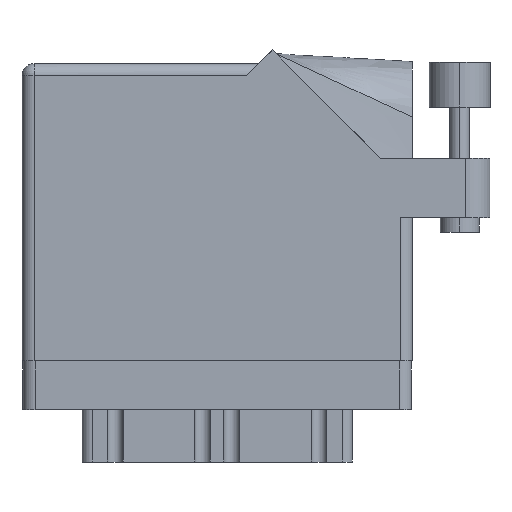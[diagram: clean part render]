
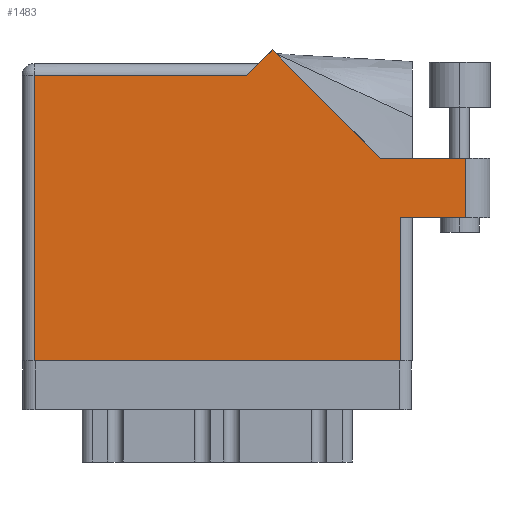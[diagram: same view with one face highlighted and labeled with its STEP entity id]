
A CAD part, front view. The second image highlights one B-rep face of the part: STEP entity #1483.
In plain terms, the highlighted face is planar.
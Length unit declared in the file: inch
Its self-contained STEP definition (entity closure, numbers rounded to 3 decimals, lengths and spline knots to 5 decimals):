
#313 = ORIENTED_EDGE ( 'NONE', *, *, #32996, .T. ) ;
#760 = CARTESIAN_POINT ( 'NONE',  ( 2.41, 1.044, 0. ) ) ;
#932 = VERTEX_POINT ( 'NONE', #34504 ) ;
#1483 = ADVANCED_FACE ( 'NONE', ( #16268 ), #7638, .F. ) ;
#1508 = CARTESIAN_POINT ( 'NONE',  ( 0., 1.468, 0. ) ) ;
#2046 = CARTESIAN_POINT ( 'NONE',  ( 0.062, 0., 0. ) ) ;
#2494 = CARTESIAN_POINT ( 'NONE',  ( 2.01, 0.737, 0. ) ) ;
#2505 = EDGE_LOOP ( 'NONE', ( #14980, #20236, #18831, #3973, #25659, #313, #23713, #31068, #27965 ) ) ;
#3094 = CARTESIAN_POINT ( 'NONE',  ( 1.155, 1.468, 0. ) ) ;
#3973 = ORIENTED_EDGE ( 'NONE', *, *, #20785, .T. ) ;
#4263 = DIRECTION ( 'NONE',  ( 0., 1., 0. ) ) ;
#4968 = LINE ( 'NONE', #2046, #15368 ) ;
#6280 = VECTOR ( 'NONE', #18075, 39.37008 ) ;
#6432 = VECTOR ( 'NONE', #33864, 39.37008 ) ;
#7322 = CARTESIAN_POINT ( 'NONE',  ( 1.948, 0., 0. ) ) ;
#7638 = PLANE ( 'NONE',  #19010 ) ;
#9730 = EDGE_CURVE ( 'NONE', #15255, #17082, #21563, .T. ) ;
#10452 = CARTESIAN_POINT ( 'NONE',  ( 0.062, 1.468, 0. ) ) ;
#10572 = DIRECTION ( 'NONE',  ( -1., 0., 0. ) ) ;
#10894 = VERTEX_POINT ( 'NONE', #10452 ) ;
#11469 = VERTEX_POINT ( 'NONE', #3094 ) ;
#11742 = VECTOR ( 'NONE', #31262, 39.37008 ) ;
#11778 = LINE ( 'NONE', #11996, #6280 ) ;
#11996 = CARTESIAN_POINT ( 'NONE',  ( 1.217, 1.53, 0. ) ) ;
#12164 = EDGE_CURVE ( 'NONE', #10894, #14437, #4968, .T. ) ;
#12780 = VERTEX_POINT ( 'NONE', #24798 ) ;
#12906 = EDGE_CURVE ( 'NONE', #12954, #932, #28499, .T. ) ;
#12954 = VERTEX_POINT ( 'NONE', #7322 ) ;
#14254 = CARTESIAN_POINT ( 'NONE',  ( 1.84442, 1.044, 0. ) ) ;
#14437 = VERTEX_POINT ( 'NONE', #14606 ) ;
#14606 = CARTESIAN_POINT ( 'NONE',  ( 0.062, 0., 0. ) ) ;
#14980 = ORIENTED_EDGE ( 'NONE', *, *, #23627, .T. ) ;
#15255 = VERTEX_POINT ( 'NONE', #27231 ) ;
#15368 = VECTOR ( 'NONE', #16556, 39.37008 ) ;
#15943 = EDGE_CURVE ( 'NONE', #12780, #11469, #11778, .T. ) ;
#16048 = CARTESIAN_POINT ( 'NONE',  ( 2.285, 1.044, 0. ) ) ;
#16268 = FACE_OUTER_BOUND ( 'NONE', #2505, .T. ) ;
#16556 = DIRECTION ( 'NONE',  ( 0., -1., 0. ) ) ;
#17082 = VERTEX_POINT ( 'NONE', #32617 ) ;
#18012 = EDGE_CURVE ( 'NONE', #14437, #12954, #22919, .T. ) ;
#18075 = DIRECTION ( 'NONE',  ( -0.707, -0.707, 0. ) ) ;
#18141 = VECTOR ( 'NONE', #4263, 39.37008 ) ;
#18784 = LINE ( 'NONE', #760, #23560 ) ;
#18831 = ORIENTED_EDGE ( 'NONE', *, *, #26727, .T. ) ;
#19010 = AXIS2_PLACEMENT_3D ( 'NONE', #19623, #28229, #10572 ) ;
#19623 = CARTESIAN_POINT ( 'NONE',  ( 0., 1.53, 0. ) ) ;
#19627 = VERTEX_POINT ( 'NONE', #14254 ) ;
#19886 = LINE ( 'NONE', #20094, #30640 ) ;
#20094 = CARTESIAN_POINT ( 'NONE',  ( 1.84442, 1.044, 0. ) ) ;
#20236 = ORIENTED_EDGE ( 'NONE', *, *, #9730, .T. ) ;
#20785 = EDGE_CURVE ( 'NONE', #19627, #12780, #19886, .T. ) ;
#21563 = LINE ( 'NONE', #16048, #18141 ) ;
#22243 = CARTESIAN_POINT ( 'NONE',  ( 1.948, 0.737, 0. ) ) ;
#22919 = LINE ( 'NONE', #25665, #32606 ) ;
#23205 = VECTOR ( 'NONE', #35605, 39.37008 ) ;
#23560 = VECTOR ( 'NONE', #24475, 39.37008 ) ;
#23627 = EDGE_CURVE ( 'NONE', #932, #15255, #29729, .T. ) ;
#23713 = ORIENTED_EDGE ( 'NONE', *, *, #12164, .T. ) ;
#24475 = DIRECTION ( 'NONE',  ( -1., 0., 0. ) ) ;
#24798 = CARTESIAN_POINT ( 'NONE',  ( 1.28771, 1.60071, 0. ) ) ;
#25659 = ORIENTED_EDGE ( 'NONE', *, *, #15943, .T. ) ;
#25665 = CARTESIAN_POINT ( 'NONE',  ( 0., 0., 0. ) ) ;
#26056 = DIRECTION ( 'NONE',  ( 1., 0., 0. ) ) ;
#26727 = EDGE_CURVE ( 'NONE', #17082, #19627, #18784, .T. ) ;
#27231 = CARTESIAN_POINT ( 'NONE',  ( 2.285, 0.737, 0. ) ) ;
#27965 = ORIENTED_EDGE ( 'NONE', *, *, #12906, .T. ) ;
#28229 = DIRECTION ( 'NONE',  ( 0., 0., -1. ) ) ;
#28499 = LINE ( 'NONE', #22243, #11742 ) ;
#29729 = LINE ( 'NONE', #2494, #23205 ) ;
#30640 = VECTOR ( 'NONE', #38307, 39.37008 ) ;
#31068 = ORIENTED_EDGE ( 'NONE', *, *, #18012, .T. ) ;
#31262 = DIRECTION ( 'NONE',  ( 0., 1., 0. ) ) ;
#32606 = VECTOR ( 'NONE', #26056, 39.37008 ) ;
#32617 = CARTESIAN_POINT ( 'NONE',  ( 2.285, 1.044, 0. ) ) ;
#32996 = EDGE_CURVE ( 'NONE', #11469, #10894, #33659, .T. ) ;
#33659 = LINE ( 'NONE', #1508, #6432 ) ;
#33864 = DIRECTION ( 'NONE',  ( -1., 0., 0. ) ) ;
#34504 = CARTESIAN_POINT ( 'NONE',  ( 1.948, 0.737, 0. ) ) ;
#35605 = DIRECTION ( 'NONE',  ( 1., 0., 0. ) ) ;
#38307 = DIRECTION ( 'NONE',  ( -0.707, 0.707, 0. ) ) ;
